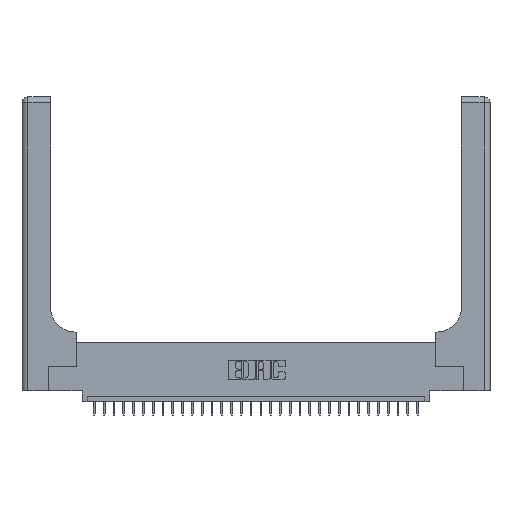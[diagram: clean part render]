
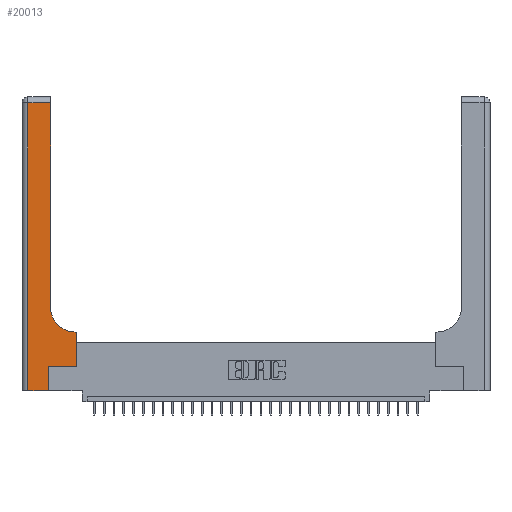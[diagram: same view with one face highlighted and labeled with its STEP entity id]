
A CAD part, top view. The second image highlights one B-rep face of the part: STEP entity #20013.
In plain terms, the highlighted planar face has unit normal (0, 0, 1).
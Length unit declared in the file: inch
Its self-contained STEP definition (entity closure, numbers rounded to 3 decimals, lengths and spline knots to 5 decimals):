
#33 = VERTEX_POINT ( 'NONE', #25167 ) ;
#434 = EDGE_CURVE ( 'NONE', #6606, #7317, #19955, .T. ) ;
#512 = ORIENTED_EDGE ( 'NONE', *, *, #23762, .T. ) ;
#1001 = VECTOR ( 'NONE', #9380, 39.37008 ) ;
#1288 = DIRECTION ( 'NONE',  ( -1., 0., 0. ) ) ;
#1491 = LINE ( 'NONE', #11405, #18406 ) ;
#1755 = DIRECTION ( 'NONE',  ( 1., 0., 0. ) ) ;
#2100 = CARTESIAN_POINT ( 'NONE',  ( 0.5585, 0.6, 0.37 ) ) ;
#2898 = EDGE_CURVE ( 'NONE', #7317, #15211, #1491, .T. ) ;
#2931 = FACE_OUTER_BOUND ( 'NONE', #19374, .T. ) ;
#3756 = CARTESIAN_POINT ( 'NONE',  ( 0.5415, 0.85, 0.37 ) ) ;
#4024 = CARTESIAN_POINT ( 'NONE',  ( 0., 0., 0.37 ) ) ;
#4078 = VERTEX_POINT ( 'NONE', #9675 ) ;
#5646 = AXIS2_PLACEMENT_3D ( 'NONE', #3756, #18551, #25988 ) ;
#6013 = ORIENTED_EDGE ( 'NONE', *, *, #23918, .T. ) ;
#6027 = ORIENTED_EDGE ( 'NONE', *, *, #27706, .T. ) ;
#6426 = VECTOR ( 'NONE', #23040, 39.37008 ) ;
#6606 = VERTEX_POINT ( 'NONE', #21582 ) ;
#6684 = CIRCLE ( 'NONE', #5646, 0.25 ) ;
#7317 = VERTEX_POINT ( 'NONE', #7482 ) ;
#7482 = CARTESIAN_POINT ( 'NONE',  ( 0.5585, 0.25, 0.37 ) ) ;
#7958 = CARTESIAN_POINT ( 'NONE',  ( 0., 2.94, 0.37 ) ) ;
#8241 = VECTOR ( 'NONE', #10367, 39.37008 ) ;
#8599 = DIRECTION ( 'NONE',  ( 0., 0., -1. ) ) ;
#9232 = VERTEX_POINT ( 'NONE', #11790 ) ;
#9380 = DIRECTION ( 'NONE',  ( 0., -1., 0. ) ) ;
#9554 = VECTOR ( 'NONE', #10553, 39.37008 ) ;
#9617 = VECTOR ( 'NONE', #1755, 39.37008 ) ;
#9675 = CARTESIAN_POINT ( 'NONE',  ( 0.06, 0., 0.37 ) ) ;
#9970 = EDGE_CURVE ( 'NONE', #33, #19202, #6684, .T. ) ;
#10119 = EDGE_CURVE ( 'NONE', #9232, #6606, #22854, .T. ) ;
#10208 = DIRECTION ( 'NONE',  ( 1., 0., 0. ) ) ;
#10367 = DIRECTION ( 'NONE',  ( 0., 1., 0. ) ) ;
#10553 = DIRECTION ( 'NONE',  ( -1., 0., 0. ) ) ;
#11405 = CARTESIAN_POINT ( 'NONE',  ( 0.5585, 0.25, 0.37 ) ) ;
#11790 = CARTESIAN_POINT ( 'NONE',  ( 0.269, 0., 0.37 ) ) ;
#11955 = VERTEX_POINT ( 'NONE', #15875 ) ;
#14008 = DIRECTION ( 'NONE',  ( 0., 1., 0. ) ) ;
#14270 = CARTESIAN_POINT ( 'NONE',  ( 0.06, 3., 0.37 ) ) ;
#14291 = ORIENTED_EDGE ( 'NONE', *, *, #434, .T. ) ;
#14449 = EDGE_CURVE ( 'NONE', #11955, #23253, #30481, .T. ) ;
#14803 = LINE ( 'NONE', #27099, #9554 ) ;
#15027 = ORIENTED_EDGE ( 'NONE', *, *, #16920, .T. ) ;
#15211 = VERTEX_POINT ( 'NONE', #2100 ) ;
#15223 = ORIENTED_EDGE ( 'NONE', *, *, #10119, .T. ) ;
#15602 = LINE ( 'NONE', #28374, #6426 ) ;
#15875 = CARTESIAN_POINT ( 'NONE',  ( 0.2915, 2.94, 0.37 ) ) ;
#16689 = LINE ( 'NONE', #14270, #1001 ) ;
#16920 = EDGE_CURVE ( 'NONE', #23253, #4078, #16689, .T. ) ;
#17352 = CARTESIAN_POINT ( 'NONE',  ( 0.269, 0.25, 0.37 ) ) ;
#18358 = PLANE ( 'NONE',  #30587 ) ;
#18406 = VECTOR ( 'NONE', #14008, 39.37008 ) ;
#18515 = ORIENTED_EDGE ( 'NONE', *, *, #14449, .T. ) ;
#18551 = DIRECTION ( 'NONE',  ( 0., 0., -1. ) ) ;
#19202 = VERTEX_POINT ( 'NONE', #28497 ) ;
#19231 = VECTOR ( 'NONE', #1288, 39.37008 ) ;
#19374 = EDGE_LOOP ( 'NONE', ( #6013, #18515, #15027, #6027, #15223, #14291, #31309, #512, #23385 ) ) ;
#19955 = LINE ( 'NONE', #17352, #26062 ) ;
#20013 = ADVANCED_FACE ( 'NONE', ( #2931 ), #18358, .F. ) ;
#20106 = CARTESIAN_POINT ( 'NONE',  ( 0.269, 0., 0.37 ) ) ;
#21582 = CARTESIAN_POINT ( 'NONE',  ( 0.269, 0.25, 0.37 ) ) ;
#22854 = LINE ( 'NONE', #20106, #8241 ) ;
#23040 = DIRECTION ( 'NONE',  ( 0., 1., 0. ) ) ;
#23253 = VERTEX_POINT ( 'NONE', #25028 ) ;
#23385 = ORIENTED_EDGE ( 'NONE', *, *, #9970, .T. ) ;
#23762 = EDGE_CURVE ( 'NONE', #15211, #33, #14803, .T. ) ;
#23918 = EDGE_CURVE ( 'NONE', #19202, #11955, #15602, .T. ) ;
#23986 = LINE ( 'NONE', #4024, #9617 ) ;
#25028 = CARTESIAN_POINT ( 'NONE',  ( 0.06, 2.94, 0.37 ) ) ;
#25167 = CARTESIAN_POINT ( 'NONE',  ( 0.5415, 0.6, 0.37 ) ) ;
#25788 = CARTESIAN_POINT ( 'NONE',  ( 0., 3., 0.37 ) ) ;
#25988 = DIRECTION ( 'NONE',  ( 1., 0., 0. ) ) ;
#26062 = VECTOR ( 'NONE', #10208, 39.37008 ) ;
#27099 = CARTESIAN_POINT ( 'NONE',  ( 0.2915, 0.6, 0.37 ) ) ;
#27706 = EDGE_CURVE ( 'NONE', #4078, #9232, #23986, .T. ) ;
#28374 = CARTESIAN_POINT ( 'NONE',  ( 0.2915, 3., 0.37 ) ) ;
#28497 = CARTESIAN_POINT ( 'NONE',  ( 0.2915, 0.85, 0.37 ) ) ;
#30481 = LINE ( 'NONE', #7958, #19231 ) ;
#30489 = DIRECTION ( 'NONE',  ( -1., 0., 0. ) ) ;
#30587 = AXIS2_PLACEMENT_3D ( 'NONE', #25788, #8599, #30489 ) ;
#31309 = ORIENTED_EDGE ( 'NONE', *, *, #2898, .T. ) ;
